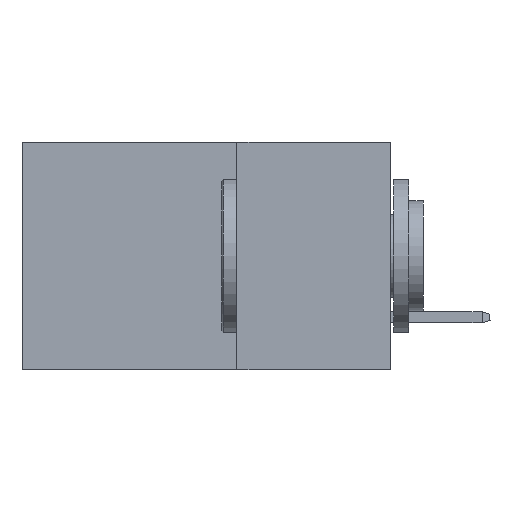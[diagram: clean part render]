
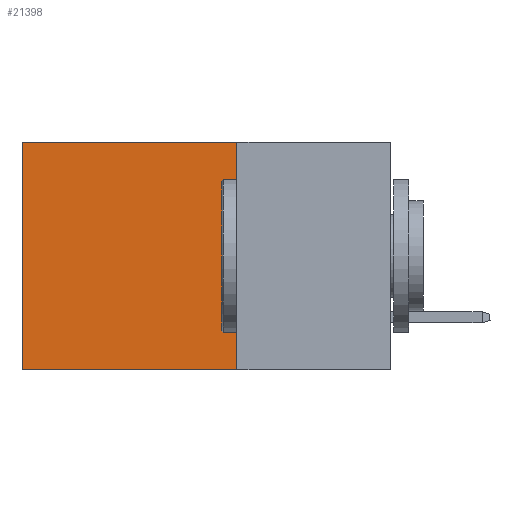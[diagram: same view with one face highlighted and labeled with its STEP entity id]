
A CAD part, left-side view. The second image highlights one B-rep face of the part: STEP entity #21398.
In plain terms, the highlighted planar face has unit normal (-1, 0, 0).
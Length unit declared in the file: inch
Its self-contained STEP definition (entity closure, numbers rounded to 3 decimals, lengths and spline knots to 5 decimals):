
#426 = CARTESIAN_POINT ( 'NONE',  ( 0.2875, 0.25, 0. ) ) ;
#1094 = DIRECTION ( 'NONE',  ( 0., 1., 0. ) ) ;
#1804 = EDGE_LOOP ( 'NONE', ( #7494, #27019, #27102, #2363 ) ) ;
#1940 = DIRECTION ( 'NONE',  ( 0., 0., -1. ) ) ;
#2363 = ORIENTED_EDGE ( 'NONE', *, *, #22643, .T. ) ;
#2775 = DIRECTION ( 'NONE',  ( 0., 0., -1. ) ) ;
#3318 = FACE_OUTER_BOUND ( 'NONE', #1804, .T. ) ;
#3449 = DIRECTION ( 'NONE',  ( 0., 1., 0. ) ) ;
#5211 = VECTOR ( 'NONE', #1940, 39.37008 ) ;
#5557 = DIRECTION ( 'NONE',  ( 0., 0., -1. ) ) ;
#5758 = CARTESIAN_POINT ( 'NONE',  ( 0.2875, 0.6, 0. ) ) ;
#6460 = VECTOR ( 'NONE', #5557, 39.37008 ) ;
#7420 = VECTOR ( 'NONE', #3449, 39.37008 ) ;
#7494 = ORIENTED_EDGE ( 'NONE', *, *, #21430, .T. ) ;
#8499 = CARTESIAN_POINT ( 'NONE',  ( 0.2875, 0.6, -0.37 ) ) ;
#9405 = DIRECTION ( 'NONE',  ( 1., 0., 0. ) ) ;
#9427 = VERTEX_POINT ( 'NONE', #8499 ) ;
#9894 = LINE ( 'NONE', #5758, #6460 ) ;
#10034 = CARTESIAN_POINT ( 'NONE',  ( 0.2875, 0.25, -0.37 ) ) ;
#13870 = LINE ( 'NONE', #24084, #5211 ) ;
#15104 = VERTEX_POINT ( 'NONE', #23666 ) ;
#18791 = VERTEX_POINT ( 'NONE', #22141 ) ;
#18935 = CARTESIAN_POINT ( 'NONE',  ( 0.2875, 0.25, 0. ) ) ;
#20571 = EDGE_CURVE ( 'NONE', #25675, #9427, #28225, .T. ) ;
#21398 = ADVANCED_FACE ( 'NONE', ( #3318 ), #26922, .F. ) ;
#21430 = EDGE_CURVE ( 'NONE', #18791, #9427, #9894, .T. ) ;
#22141 = CARTESIAN_POINT ( 'NONE',  ( 0.2875, 0.6, 0. ) ) ;
#22643 = EDGE_CURVE ( 'NONE', #15104, #18791, #26354, .T. ) ;
#23663 = EDGE_CURVE ( 'NONE', #15104, #25675, #13870, .T. ) ;
#23666 = CARTESIAN_POINT ( 'NONE',  ( 0.2875, 0.25, 0. ) ) ;
#24003 = AXIS2_PLACEMENT_3D ( 'NONE', #426, #9405, #2775 ) ;
#24084 = CARTESIAN_POINT ( 'NONE',  ( 0.2875, 0.25, 0. ) ) ;
#25675 = VERTEX_POINT ( 'NONE', #10034 ) ;
#25802 = VECTOR ( 'NONE', #1094, 39.37008 ) ;
#26354 = LINE ( 'NONE', #18935, #7420 ) ;
#26922 = PLANE ( 'NONE',  #24003 ) ;
#27019 = ORIENTED_EDGE ( 'NONE', *, *, #20571, .F. ) ;
#27102 = ORIENTED_EDGE ( 'NONE', *, *, #23663, .F. ) ;
#27551 = CARTESIAN_POINT ( 'NONE',  ( 0.2875, 0.25, -0.37 ) ) ;
#28225 = LINE ( 'NONE', #27551, #25802 ) ;
